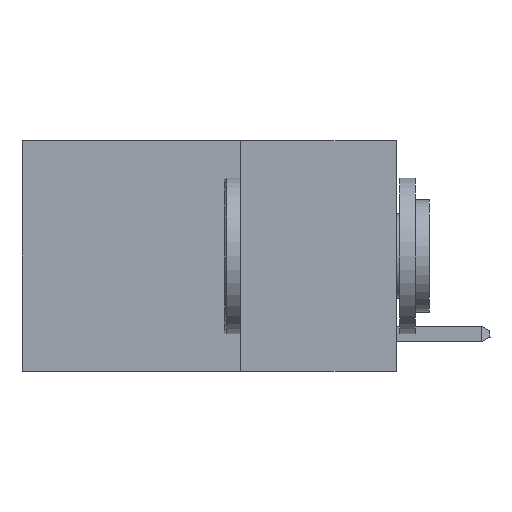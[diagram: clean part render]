
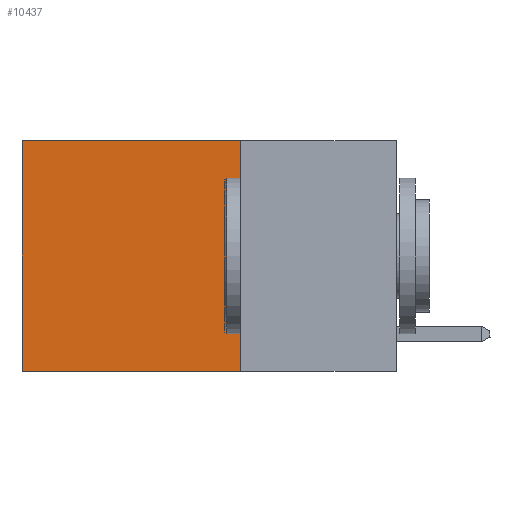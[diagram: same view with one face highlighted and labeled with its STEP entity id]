
A CAD part, left-side view. The second image highlights one B-rep face of the part: STEP entity #10437.
In plain terms, the highlighted planar face has unit normal (-1, 0, 0).
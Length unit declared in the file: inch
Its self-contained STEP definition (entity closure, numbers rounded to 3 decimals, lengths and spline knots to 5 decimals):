
#276 = VERTEX_POINT ( 'NONE', #963 ) ;
#315 = DIRECTION ( 'NONE',  ( 0., 0., -1. ) ) ;
#588 = DIRECTION ( 'NONE',  ( 0., 1., 0. ) ) ;
#963 = CARTESIAN_POINT ( 'NONE',  ( 0.2625, 0.6, 0. ) ) ;
#1316 = CARTESIAN_POINT ( 'NONE',  ( 0.2625, 0.25, 0. ) ) ;
#1372 = EDGE_LOOP ( 'NONE', ( #11768, #4330, #6901, #10159 ) ) ;
#1504 = LINE ( 'NONE', #7033, #8347 ) ;
#2169 = PLANE ( 'NONE',  #11245 ) ;
#2359 = FACE_OUTER_BOUND ( 'NONE', #1372, .T. ) ;
#2488 = VECTOR ( 'NONE', #6847, 39.37008 ) ;
#2598 = LINE ( 'NONE', #9888, #6496 ) ;
#4127 = CARTESIAN_POINT ( 'NONE',  ( 0.2625, 0.25, 0. ) ) ;
#4330 = ORIENTED_EDGE ( 'NONE', *, *, #9341, .F. ) ;
#5050 = CARTESIAN_POINT ( 'NONE',  ( 0.2625, 0.25, 0. ) ) ;
#5386 = EDGE_CURVE ( 'NONE', #276, #11273, #2598, .T. ) ;
#5571 = CARTESIAN_POINT ( 'NONE',  ( 0.2625, 0.6, -0.37 ) ) ;
#6496 = VECTOR ( 'NONE', #10136, 39.37008 ) ;
#6792 = EDGE_CURVE ( 'NONE', #11760, #8761, #8773, .T. ) ;
#6847 = DIRECTION ( 'NONE',  ( 0., 1., 0. ) ) ;
#6901 = ORIENTED_EDGE ( 'NONE', *, *, #6792, .F. ) ;
#7033 = CARTESIAN_POINT ( 'NONE',  ( 0.2625, 0.25, -0.37 ) ) ;
#7502 = VECTOR ( 'NONE', #315, 39.37008 ) ;
#7843 = DIRECTION ( 'NONE',  ( 1., 0., 0. ) ) ;
#8347 = VECTOR ( 'NONE', #588, 39.37008 ) ;
#8761 = VERTEX_POINT ( 'NONE', #11648 ) ;
#8773 = LINE ( 'NONE', #4127, #7502 ) ;
#9173 = EDGE_CURVE ( 'NONE', #11760, #276, #9646, .T. ) ;
#9312 = CARTESIAN_POINT ( 'NONE',  ( 0.2625, 0.25, 0. ) ) ;
#9341 = EDGE_CURVE ( 'NONE', #8761, #11273, #1504, .T. ) ;
#9646 = LINE ( 'NONE', #1316, #2488 ) ;
#9888 = CARTESIAN_POINT ( 'NONE',  ( 0.2625, 0.6, 0. ) ) ;
#10136 = DIRECTION ( 'NONE',  ( 0., 0., -1. ) ) ;
#10159 = ORIENTED_EDGE ( 'NONE', *, *, #9173, .T. ) ;
#10437 = ADVANCED_FACE ( 'NONE', ( #2359 ), #2169, .F. ) ;
#10512 = DIRECTION ( 'NONE',  ( 0., 0., -1. ) ) ;
#11245 = AXIS2_PLACEMENT_3D ( 'NONE', #5050, #7843, #10512 ) ;
#11273 = VERTEX_POINT ( 'NONE', #5571 ) ;
#11648 = CARTESIAN_POINT ( 'NONE',  ( 0.2625, 0.25, -0.37 ) ) ;
#11760 = VERTEX_POINT ( 'NONE', #9312 ) ;
#11768 = ORIENTED_EDGE ( 'NONE', *, *, #5386, .T. ) ;
